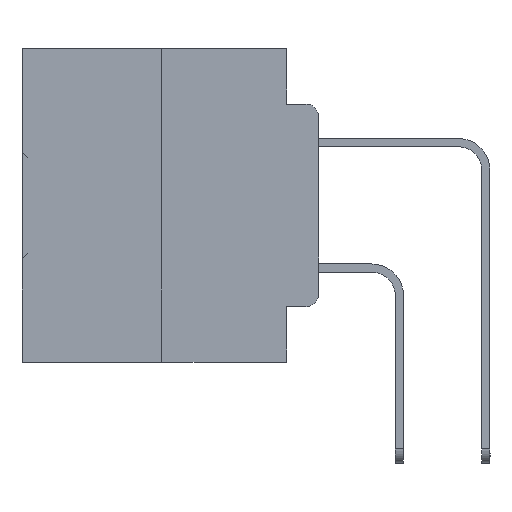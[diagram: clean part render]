
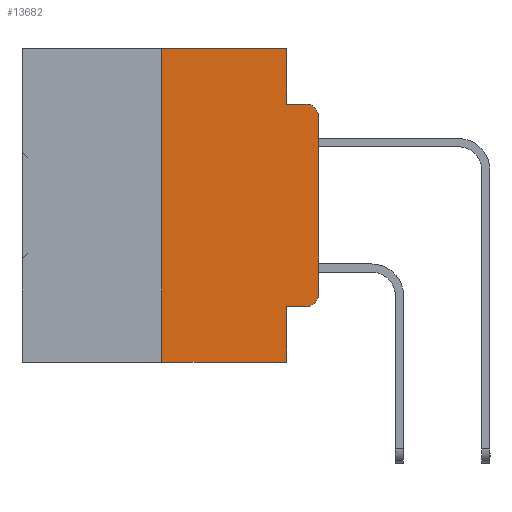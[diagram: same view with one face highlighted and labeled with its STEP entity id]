
A CAD part, left-side view. The second image highlights one B-rep face of the part: STEP entity #13682.
In plain terms, the highlighted planar face has unit normal (-1, 0, 0).
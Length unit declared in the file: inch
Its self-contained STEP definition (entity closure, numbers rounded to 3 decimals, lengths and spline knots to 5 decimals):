
#107 = LINE ( 'NONE', #9009, #15599 ) ;
#302 = DIRECTION ( 'NONE',  ( 0., 0., -1. ) ) ;
#306 = DIRECTION ( 'NONE',  ( 0., 0., -1. ) ) ;
#478 = LINE ( 'NONE', #35023, #21585 ) ;
#2150 = VECTOR ( 'NONE', #16564, 39.37008 ) ;
#2433 = ORIENTED_EDGE ( 'NONE', *, *, #12351, .F. ) ;
#3155 = CARTESIAN_POINT ( 'NONE',  ( 0., 0.473, 0. ) ) ;
#3317 = DIRECTION ( 'NONE',  ( 0., 0., -1. ) ) ;
#3654 = CARTESIAN_POINT ( 'NONE',  ( 0., 0.051, -0.4115 ) ) ;
#3674 = VERTEX_POINT ( 'NONE', #18480 ) ;
#4090 = CARTESIAN_POINT ( 'NONE',  ( 0., 0.02, -0.3915 ) ) ;
#4380 = CARTESIAN_POINT ( 'NONE',  ( 0., 0.051, -0.0885 ) ) ;
#4527 = ORIENTED_EDGE ( 'NONE', *, *, #18526, .T. ) ;
#4632 = EDGE_CURVE ( 'NONE', #16444, #3674, #18348, .T. ) ;
#5473 = DIRECTION ( 'NONE',  ( 0., 0., 1. ) ) ;
#5985 = DIRECTION ( 'NONE',  ( -1., 0., 0. ) ) ;
#6500 = EDGE_CURVE ( 'NONE', #25600, #13693, #28635, .T. ) ;
#6572 = CARTESIAN_POINT ( 'NONE',  ( 0., 0.02, -0.1085 ) ) ;
#7115 = ORIENTED_EDGE ( 'NONE', *, *, #19177, .T. ) ;
#7343 = DIRECTION ( 'NONE',  ( -1., 0., 0. ) ) ;
#8265 = VECTOR ( 'NONE', #5473, 39.37008 ) ;
#8456 = VERTEX_POINT ( 'NONE', #4380 ) ;
#8639 = AXIS2_PLACEMENT_3D ( 'NONE', #3155, #26159, #302 ) ;
#9009 = CARTESIAN_POINT ( 'NONE',  ( 0., 0.051, 0. ) ) ;
#10161 = VERTEX_POINT ( 'NONE', #18316 ) ;
#10605 = CARTESIAN_POINT ( 'NONE',  ( 0., 0., 0. ) ) ;
#10720 = CARTESIAN_POINT ( 'NONE',  ( 0., 0.25, 0. ) ) ;
#11849 = FACE_OUTER_BOUND ( 'NONE', #35360, .T. ) ;
#12351 = EDGE_CURVE ( 'NONE', #8456, #16454, #15388, .T. ) ;
#12872 = ORIENTED_EDGE ( 'NONE', *, *, #23132, .F. ) ;
#12921 = CARTESIAN_POINT ( 'NONE',  ( 0., 0.051, -0.0885 ) ) ;
#13220 = VECTOR ( 'NONE', #33629, 39.37008 ) ;
#13430 = LINE ( 'NONE', #10605, #8265 ) ;
#13682 = ADVANCED_FACE ( 'NONE', ( #11849 ), #35220, .F. ) ;
#13693 = VERTEX_POINT ( 'NONE', #18060 ) ;
#14160 = CARTESIAN_POINT ( 'NONE',  ( 0., 0., -0.1085 ) ) ;
#15388 = LINE ( 'NONE', #12921, #27219 ) ;
#15599 = VECTOR ( 'NONE', #3317, 39.37008 ) ;
#16444 = VERTEX_POINT ( 'NONE', #3654 ) ;
#16454 = VERTEX_POINT ( 'NONE', #26112 ) ;
#16564 = DIRECTION ( 'NONE',  ( 0., 0., 1. ) ) ;
#16940 = LINE ( 'NONE', #10720, #2150 ) ;
#17605 = AXIS2_PLACEMENT_3D ( 'NONE', #6572, #5985, #306 ) ;
#17696 = CARTESIAN_POINT ( 'NONE',  ( 0., 0.051, 0. ) ) ;
#18060 = CARTESIAN_POINT ( 'NONE',  ( 0., 0.051, -0.5 ) ) ;
#18066 = DIRECTION ( 'NONE',  ( 0., 0., -1. ) ) ;
#18258 = VECTOR ( 'NONE', #22595, 39.37008 ) ;
#18316 = CARTESIAN_POINT ( 'NONE',  ( 0., 0.25, 0. ) ) ;
#18348 = LINE ( 'NONE', #29849, #13220 ) ;
#18480 = CARTESIAN_POINT ( 'NONE',  ( 0., 0.02, -0.4115 ) ) ;
#18526 = EDGE_CURVE ( 'NONE', #37275, #22675, #13430, .T. ) ;
#19177 = EDGE_CURVE ( 'NONE', #3674, #37275, #20283, .T. ) ;
#19206 = ORIENTED_EDGE ( 'NONE', *, *, #25342, .F. ) ;
#20018 = CIRCLE ( 'NONE', #17605, 0.02 ) ;
#20283 = CIRCLE ( 'NONE', #20876, 0.02 ) ;
#20664 = CARTESIAN_POINT ( 'NONE',  ( 0., 0., -0.3915 ) ) ;
#20808 = LINE ( 'NONE', #35350, #20852 ) ;
#20852 = VECTOR ( 'NONE', #23639, 39.37008 ) ;
#20876 = AXIS2_PLACEMENT_3D ( 'NONE', #4090, #7343, #18066 ) ;
#21272 = EDGE_CURVE ( 'NONE', #25600, #10161, #16940, .T. ) ;
#21585 = VECTOR ( 'NONE', #29531, 39.37008 ) ;
#22331 = ORIENTED_EDGE ( 'NONE', *, *, #30920, .T. ) ;
#22595 = DIRECTION ( 'NONE',  ( 0., -1., 0. ) ) ;
#22675 = VERTEX_POINT ( 'NONE', #14160 ) ;
#23132 = EDGE_CURVE ( 'NONE', #16444, #13693, #20808, .T. ) ;
#23639 = DIRECTION ( 'NONE',  ( 0., 0., -1. ) ) ;
#24526 = ORIENTED_EDGE ( 'NONE', *, *, #4632, .T. ) ;
#25061 = ORIENTED_EDGE ( 'NONE', *, *, #21272, .F. ) ;
#25279 = EDGE_CURVE ( 'NONE', #10161, #28008, #478, .T. ) ;
#25342 = EDGE_CURVE ( 'NONE', #28008, #8456, #107, .T. ) ;
#25577 = ORIENTED_EDGE ( 'NONE', *, *, #25279, .F. ) ;
#25600 = VERTEX_POINT ( 'NONE', #28564 ) ;
#26112 = CARTESIAN_POINT ( 'NONE',  ( 0., 0.02, -0.0885 ) ) ;
#26159 = DIRECTION ( 'NONE',  ( 1., 0., 0. ) ) ;
#27219 = VECTOR ( 'NONE', #33108, 39.37008 ) ;
#27224 = ORIENTED_EDGE ( 'NONE', *, *, #6500, .T. ) ;
#28008 = VERTEX_POINT ( 'NONE', #17696 ) ;
#28564 = CARTESIAN_POINT ( 'NONE',  ( 0., 0.25, -0.5 ) ) ;
#28635 = LINE ( 'NONE', #34320, #18258 ) ;
#29531 = DIRECTION ( 'NONE',  ( 0., -1., 0. ) ) ;
#29849 = CARTESIAN_POINT ( 'NONE',  ( 0., 0.051, -0.4115 ) ) ;
#30920 = EDGE_CURVE ( 'NONE', #22675, #16454, #20018, .T. ) ;
#33108 = DIRECTION ( 'NONE',  ( 0., -1., 0. ) ) ;
#33629 = DIRECTION ( 'NONE',  ( 0., -1., 0. ) ) ;
#34320 = CARTESIAN_POINT ( 'NONE',  ( 0., 0.473, -0.5 ) ) ;
#35023 = CARTESIAN_POINT ( 'NONE',  ( 0., 0.473, 0. ) ) ;
#35220 = PLANE ( 'NONE',  #8639 ) ;
#35350 = CARTESIAN_POINT ( 'NONE',  ( 0., 0.051, 0. ) ) ;
#35360 = EDGE_LOOP ( 'NONE', ( #4527, #22331, #2433, #19206, #25577, #25061, #27224, #12872, #24526, #7115 ) ) ;
#37275 = VERTEX_POINT ( 'NONE', #20664 ) ;
